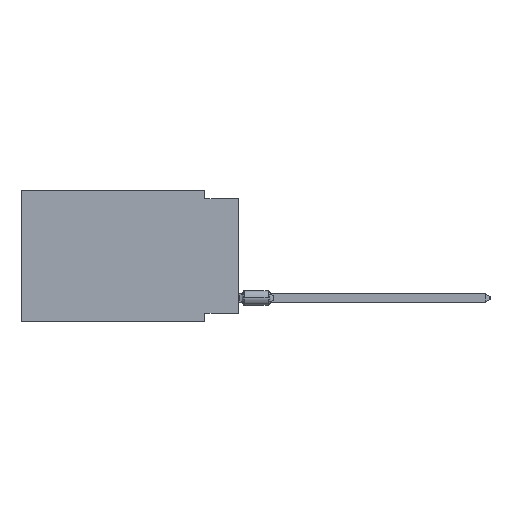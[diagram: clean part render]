
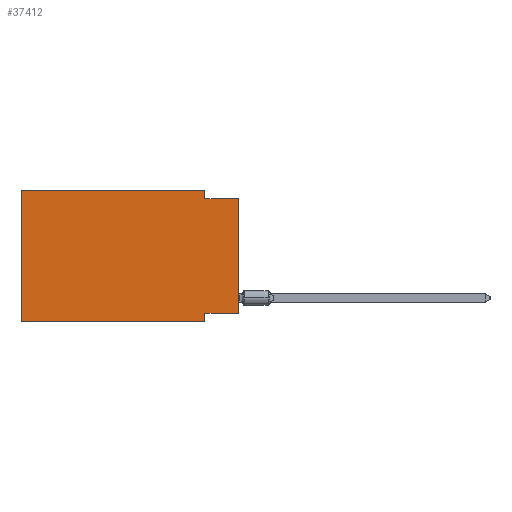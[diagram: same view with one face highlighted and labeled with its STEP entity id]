
A CAD part, left-side view. The second image highlights one B-rep face of the part: STEP entity #37412.
In plain terms, the highlighted planar face has unit normal (-1, 0, 0).
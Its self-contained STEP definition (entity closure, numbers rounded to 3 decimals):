
#824 = AXIS2_PLACEMENT_3D ( 'NONE', #17940, #57026, #56588 ) ;
#1630 = ORIENTED_EDGE ( 'NONE', *, *, #58860, .T. ) ;
#2651 = VECTOR ( 'NONE', #13892, 1000. ) ;
#3045 = CARTESIAN_POINT ( 'NONE',  ( 0., 0., -9.271 ) ) ;
#8279 = VECTOR ( 'NONE', #83549, 1000. ) ;
#8626 = VERTEX_POINT ( 'NONE', #68212 ) ;
#10439 = VERTEX_POINT ( 'NONE', #27639 ) ;
#10748 = VECTOR ( 'NONE', #29578, 1000. ) ;
#13480 = LINE ( 'NONE', #79334, #2651 ) ;
#13892 = DIRECTION ( 'NONE',  ( 0., 0., 1. ) ) ;
#14432 = VECTOR ( 'NONE', #58376, 1000. ) ;
#15320 = CARTESIAN_POINT ( 'NONE',  ( 0., 16.383, 0. ) ) ;
#16438 = LINE ( 'NONE', #47867, #82292 ) ;
#17004 = ORIENTED_EDGE ( 'NONE', *, *, #52067, .F. ) ;
#17940 = CARTESIAN_POINT ( 'NONE',  ( 0., 16.383, 0. ) ) ;
#18545 = CARTESIAN_POINT ( 'NONE',  ( 0., 0., -9.271 ) ) ;
#18750 = EDGE_CURVE ( 'NONE', #45279, #80428, #74027, .T. ) ;
#19142 = CARTESIAN_POINT ( 'NONE',  ( 0., 0., -0.635 ) ) ;
#19955 = LINE ( 'NONE', #19142, #43047 ) ;
#20689 = ORIENTED_EDGE ( 'NONE', *, *, #79524, .F. ) ;
#21776 = CARTESIAN_POINT ( 'NONE',  ( 0., 16.383, -9.906 ) ) ;
#22055 = EDGE_CURVE ( 'NONE', #74908, #10439, #13480, .T. ) ;
#24628 = ORIENTED_EDGE ( 'NONE', *, *, #36220, .F. ) ;
#24671 = LINE ( 'NONE', #52236, #55294 ) ;
#27639 = CARTESIAN_POINT ( 'NONE',  ( 0., 0., -0.635 ) ) ;
#28780 = VERTEX_POINT ( 'NONE', #21776 ) ;
#29578 = DIRECTION ( 'NONE',  ( 0., 0., -1. ) ) ;
#29733 = VERTEX_POINT ( 'NONE', #69050 ) ;
#32513 = LINE ( 'NONE', #18545, #8279 ) ;
#34525 = EDGE_LOOP ( 'NONE', ( #43570, #79468, #20689, #71302, #17004, #1630, #53237, #24628 ) ) ;
#36220 = EDGE_CURVE ( 'NONE', #74908, #29733, #32513, .T. ) ;
#37412 = ADVANCED_FACE ( 'NONE', ( #56168 ), #82109, .F. ) ;
#43047 = VECTOR ( 'NONE', #63775, 1000. ) ;
#43570 = ORIENTED_EDGE ( 'NONE', *, *, #22055, .T. ) ;
#45279 = VERTEX_POINT ( 'NONE', #15320 ) ;
#47867 = CARTESIAN_POINT ( 'NONE',  ( 0., 2.54, 0. ) ) ;
#48489 = CARTESIAN_POINT ( 'NONE',  ( 0., 16.383, 0. ) ) ;
#48701 = CARTESIAN_POINT ( 'NONE',  ( 0., 2.54, -9.906 ) ) ;
#48916 = CARTESIAN_POINT ( 'NONE',  ( 0., 2.54, 0. ) ) ;
#52067 = EDGE_CURVE ( 'NONE', #28780, #45279, #70308, .T. ) ;
#52236 = CARTESIAN_POINT ( 'NONE',  ( 0., 16.383, -9.906 ) ) ;
#53237 = ORIENTED_EDGE ( 'NONE', *, *, #55375, .F. ) ;
#55294 = VECTOR ( 'NONE', #70566, 1000. ) ;
#55375 = EDGE_CURVE ( 'NONE', #29733, #8626, #68272, .T. ) ;
#56168 = FACE_OUTER_BOUND ( 'NONE', #34525, .T. ) ;
#56588 = DIRECTION ( 'NONE',  ( 0., 0., -1. ) ) ;
#57026 = DIRECTION ( 'NONE',  ( 1., 0., 0. ) ) ;
#58376 = DIRECTION ( 'NONE',  ( 0., 0., 1. ) ) ;
#58849 = EDGE_CURVE ( 'NONE', #61091, #10439, #19955, .T. ) ;
#58860 = EDGE_CURVE ( 'NONE', #28780, #8626, #24671, .T. ) ;
#61091 = VERTEX_POINT ( 'NONE', #67740 ) ;
#61697 = DIRECTION ( 'NONE',  ( 0., -1., 0. ) ) ;
#63775 = DIRECTION ( 'NONE',  ( 0., -1., 0. ) ) ;
#67740 = CARTESIAN_POINT ( 'NONE',  ( 0., 2.54, -0.635 ) ) ;
#67862 = DIRECTION ( 'NONE',  ( 0., 0., -1. ) ) ;
#68212 = CARTESIAN_POINT ( 'NONE',  ( 0., 2.54, -9.906 ) ) ;
#68272 = LINE ( 'NONE', #48701, #10748 ) ;
#69050 = CARTESIAN_POINT ( 'NONE',  ( 0., 2.54, -9.271 ) ) ;
#70308 = LINE ( 'NONE', #70726, #14432 ) ;
#70566 = DIRECTION ( 'NONE',  ( 0., -1., 0. ) ) ;
#70726 = CARTESIAN_POINT ( 'NONE',  ( 0., 16.383, 0. ) ) ;
#71302 = ORIENTED_EDGE ( 'NONE', *, *, #18750, .F. ) ;
#74027 = LINE ( 'NONE', #48489, #76918 ) ;
#74908 = VERTEX_POINT ( 'NONE', #3045 ) ;
#76918 = VECTOR ( 'NONE', #61697, 1000. ) ;
#79334 = CARTESIAN_POINT ( 'NONE',  ( 0., 0., 0. ) ) ;
#79468 = ORIENTED_EDGE ( 'NONE', *, *, #58849, .F. ) ;
#79524 = EDGE_CURVE ( 'NONE', #80428, #61091, #16438, .T. ) ;
#80428 = VERTEX_POINT ( 'NONE', #48916 ) ;
#82109 = PLANE ( 'NONE',  #824 ) ;
#82292 = VECTOR ( 'NONE', #67862, 1000. ) ;
#83549 = DIRECTION ( 'NONE',  ( 0., 1., 0. ) ) ;
